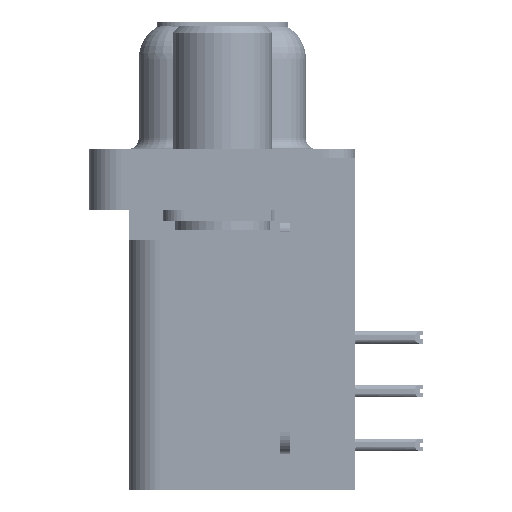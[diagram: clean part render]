
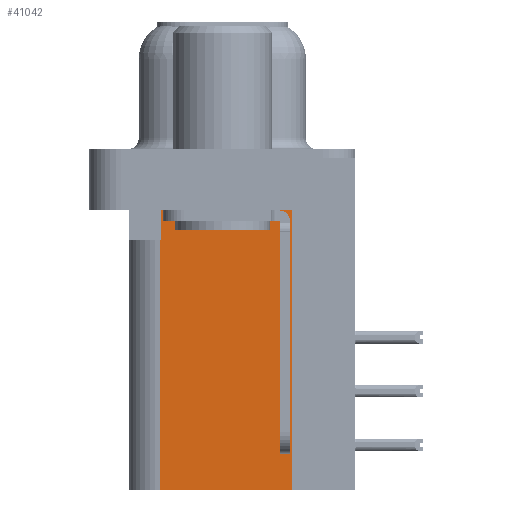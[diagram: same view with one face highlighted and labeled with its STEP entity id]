
A CAD part, left-side view. The second image highlights one B-rep face of the part: STEP entity #41042.
In plain terms, the highlighted planar face has unit normal (-1, 0, 0).
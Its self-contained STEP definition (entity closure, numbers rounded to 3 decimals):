
#779 = EDGE_CURVE ( 'NONE', #36809, #25348, #23286, .T. ) ;
#1517 = CARTESIAN_POINT ( 'NONE',  ( 3.7, 0., -3.9 ) ) ;
#2248 = LINE ( 'NONE', #22872, #10510 ) ;
#2353 = LINE ( 'NONE', #1517, #19772 ) ;
#3274 = LINE ( 'NONE', #39935, #28875 ) ;
#4440 = LINE ( 'NONE', #25997, #40350 ) ;
#5025 = DIRECTION ( 'NONE',  ( 0., 1., 0. ) ) ;
#5145 = EDGE_CURVE ( 'NONE', #24309, #36809, #4440, .T. ) ;
#6548 = CARTESIAN_POINT ( 'NONE',  ( 3.7, 2.925, -15.7 ) ) ;
#7219 = EDGE_CURVE ( 'NONE', #24309, #21533, #3274, .T. ) ;
#7359 = DIRECTION ( 'NONE',  ( 1., 0., 0. ) ) ;
#7784 = CARTESIAN_POINT ( 'NONE',  ( 3.7, 2.925, -15.7 ) ) ;
#8888 = ORIENTED_EDGE ( 'NONE', *, *, #5145, .F. ) ;
#10510 = VECTOR ( 'NONE', #26364, 1000. ) ;
#10996 = CARTESIAN_POINT ( 'NONE',  ( 3.7, -3.295, -2.5 ) ) ;
#12337 = VERTEX_POINT ( 'NONE', #44631 ) ;
#13351 = VERTEX_POINT ( 'NONE', #37105 ) ;
#14035 = VECTOR ( 'NONE', #36334, 1000. ) ;
#15990 = EDGE_LOOP ( 'NONE', ( #18078, #25856, #40853, #19866, #8888, #35868 ) ) ;
#18078 = ORIENTED_EDGE ( 'NONE', *, *, #22638, .T. ) ;
#18864 = CARTESIAN_POINT ( 'NONE',  ( 3.7, 2.895, -3.9 ) ) ;
#19033 = DIRECTION ( 'NONE',  ( 0., 0., 1. ) ) ;
#19459 = EDGE_CURVE ( 'NONE', #12337, #13351, #38979, .T. ) ;
#19772 = VECTOR ( 'NONE', #5025, 1000. ) ;
#19866 = ORIENTED_EDGE ( 'NONE', *, *, #779, .F. ) ;
#20438 = VECTOR ( 'NONE', #22394, 1000. ) ;
#21533 = VERTEX_POINT ( 'NONE', #10996 ) ;
#22394 = DIRECTION ( 'NONE',  ( 0., 0., -1. ) ) ;
#22638 = EDGE_CURVE ( 'NONE', #21533, #12337, #2248, .T. ) ;
#22872 = CARTESIAN_POINT ( 'NONE',  ( 3.7, -3.295, -2.5 ) ) ;
#23286 = LINE ( 'NONE', #6548, #14035 ) ;
#24309 = VERTEX_POINT ( 'NONE', #26795 ) ;
#25348 = VERTEX_POINT ( 'NONE', #28996 ) ;
#25835 = EDGE_CURVE ( 'NONE', #13351, #25348, #2353, .T. ) ;
#25856 = ORIENTED_EDGE ( 'NONE', *, *, #19459, .T. ) ;
#25997 = CARTESIAN_POINT ( 'NONE',  ( 3.7, -3.295, -15.7 ) ) ;
#26364 = DIRECTION ( 'NONE',  ( 0., 1., 0. ) ) ;
#26795 = CARTESIAN_POINT ( 'NONE',  ( 3.7, -3.295, -15.7 ) ) ;
#28200 = PLANE ( 'NONE',  #44797 ) ;
#28875 = VECTOR ( 'NONE', #19033, 1000. ) ;
#28996 = CARTESIAN_POINT ( 'NONE',  ( 3.7, 2.925, -3.9 ) ) ;
#31685 = DIRECTION ( 'NONE',  ( 0., 1., 0. ) ) ;
#32883 = DIRECTION ( 'NONE',  ( 0., 1., 0. ) ) ;
#33001 = FACE_OUTER_BOUND ( 'NONE', #15990, .T. ) ;
#35868 = ORIENTED_EDGE ( 'NONE', *, *, #7219, .T. ) ;
#36334 = DIRECTION ( 'NONE',  ( 0., 0., 1. ) ) ;
#36809 = VERTEX_POINT ( 'NONE', #7784 ) ;
#37105 = CARTESIAN_POINT ( 'NONE',  ( 3.7, 2.895, -3.9 ) ) ;
#38509 = CARTESIAN_POINT ( 'NONE',  ( 3.7, -3.295, -15.7 ) ) ;
#38979 = LINE ( 'NONE', #18864, #20438 ) ;
#39935 = CARTESIAN_POINT ( 'NONE',  ( 3.7, -3.295, -15.7 ) ) ;
#40350 = VECTOR ( 'NONE', #32883, 1000. ) ;
#40853 = ORIENTED_EDGE ( 'NONE', *, *, #25835, .T. ) ;
#41042 = ADVANCED_FACE ( 'NONE', ( #33001 ), #28200, .F. ) ;
#44631 = CARTESIAN_POINT ( 'NONE',  ( 3.7, 2.895, -2.5 ) ) ;
#44797 = AXIS2_PLACEMENT_3D ( 'NONE', #38509, #7359, #31685 ) ;
